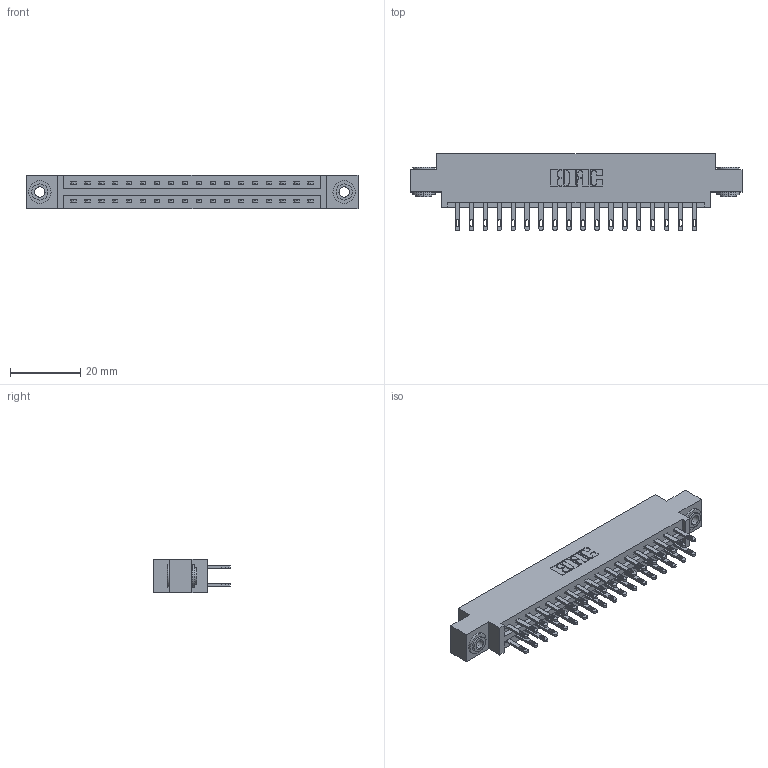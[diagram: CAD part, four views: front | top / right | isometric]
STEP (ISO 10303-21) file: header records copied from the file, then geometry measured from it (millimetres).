
FILE_DESCRIPTION (( 'STEP AP203' ), '1' );
FILE_NAME ('887-036-500-803.STEP', '2020-09-20T22:23:22', ( '' ), ( '' ), 'SwSTEP 2.0', 'SolidWorks 2020', '' );
FILE_SCHEMA (( 'CONFIG_CONTROL_DESIGN' ));
Length unit declared in the file: inch
Products named in the file (4): 887-036-500-803; 837 Part_0.170 Offset - 0.156 Dia-TH; 345-250-002_345-250-002-102; 345-292-001_345-293-100
Assembly tree (39 placements, depth 2):
  887-036-500-803
    837 Part_0.170 Offset - 0.156 Dia-TH
    345-292-001_345-293-100  x36
    345-250-002_345-250-002-102  x2
Bounding box: 94.34 x 21.85 x 9.4 mm (x, y, z)
Volume: 9634.3 mm3; surface area: 11390.1 mm2
Topology: 39 solids, 39 shells, 1956 faces, 5907 edges, 3934 vertices
Faces by surface type: plane 1236, cylinder 712, cone 8
Entity records: 17772 total; most frequent: CARTESIAN_POINT 2989, ORIENTED_EDGE 2918, DIRECTION 2621, EDGE_CURVE 1459, VECTOR 1303, LINE 1303, VERTEX_POINT 970, AXIS2_PLACEMENT_3D 659
